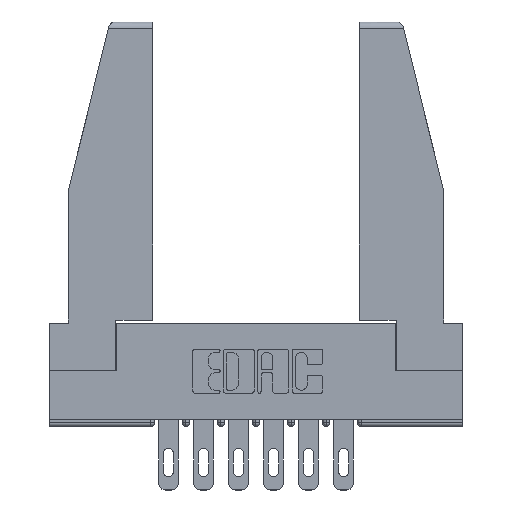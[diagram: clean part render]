
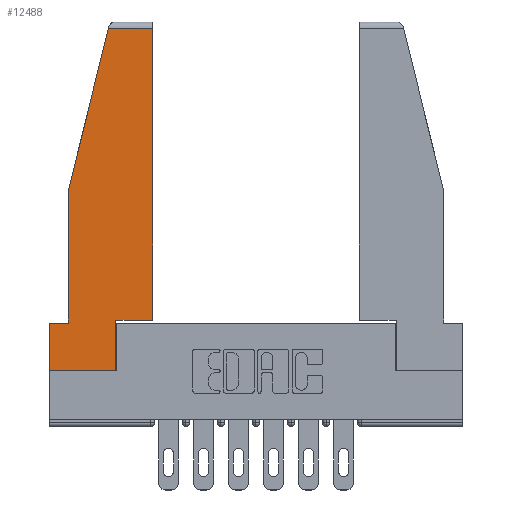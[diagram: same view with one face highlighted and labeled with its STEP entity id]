
A CAD part, top view. The second image highlights one B-rep face of the part: STEP entity #12488.
In plain terms, the highlighted planar face has unit normal (0, 0, 1).
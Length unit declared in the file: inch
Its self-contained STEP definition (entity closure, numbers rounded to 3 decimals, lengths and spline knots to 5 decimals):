
#52 = ORIENTED_EDGE ( 'NONE', *, *, #7661, .T. ) ;
#770 = LINE ( 'NONE', #2543, #12000 ) ;
#775 = DIRECTION ( 'NONE',  ( -1., 0., 0. ) ) ;
#874 = VECTOR ( 'NONE', #993, 39.37008 ) ;
#993 = DIRECTION ( 'NONE',  ( -0.239, -0.971, 0. ) ) ;
#1558 = VECTOR ( 'NONE', #3372, 39.37008 ) ;
#1620 = LINE ( 'NONE', #3783, #2023 ) ;
#1683 = DIRECTION ( 'NONE',  ( -1., 0., 0. ) ) ;
#1818 = DIRECTION ( 'NONE',  ( 1., 0., 0. ) ) ;
#1853 = CARTESIAN_POINT ( 'NONE',  ( 0., 0.21, 0. ) ) ;
#1905 = CARTESIAN_POINT ( 'NONE',  ( 0.271, 1.55, 0. ) ) ;
#2023 = VECTOR ( 'NONE', #9506, 39.37008 ) ;
#2178 = DIRECTION ( 'NONE',  ( 1., 0., 0. ) ) ;
#2543 = CARTESIAN_POINT ( 'NONE',  ( 0., 1.52, 0. ) ) ;
#2686 = ORIENTED_EDGE ( 'NONE', *, *, #4684, .T. ) ;
#2823 = CARTESIAN_POINT ( 'NONE',  ( 0.461, 1.52, 0. ) ) ;
#2955 = EDGE_CURVE ( 'NONE', #8437, #8369, #1620, .T. ) ;
#3372 = DIRECTION ( 'NONE',  ( 0., -1., 0. ) ) ;
#3496 = DIRECTION ( 'NONE',  ( 0., 1., 0. ) ) ;
#3629 = CARTESIAN_POINT ( 'NONE',  ( 0.461, 0.223, 0. ) ) ;
#3783 = CARTESIAN_POINT ( 'NONE',  ( 0.297, 0., 0. ) ) ;
#3878 = ORIENTED_EDGE ( 'NONE', *, *, #6867, .T. ) ;
#3941 = EDGE_CURVE ( 'NONE', #8189, #4542, #11826, .T. ) ;
#3943 = VERTEX_POINT ( 'NONE', #7784 ) ;
#4056 = EDGE_LOOP ( 'NONE', ( #52, #3878, #8968, #9953, #10837, #12380, #4109, #5168, #2686 ) ) ;
#4086 = EDGE_CURVE ( 'NONE', #3943, #8437, #10167, .T. ) ;
#4109 = ORIENTED_EDGE ( 'NONE', *, *, #4086, .T. ) ;
#4298 = LINE ( 'NONE', #7289, #1558 ) ;
#4358 = VERTEX_POINT ( 'NONE', #9883 ) ;
#4450 = CARTESIAN_POINT ( 'NONE',  ( 0.461, 0.223, 0. ) ) ;
#4542 = VERTEX_POINT ( 'NONE', #10339 ) ;
#4684 = EDGE_CURVE ( 'NONE', #8369, #11536, #12497, .T. ) ;
#4764 = CARTESIAN_POINT ( 'NONE',  ( 0.297, 0.223, 0. ) ) ;
#4903 = CARTESIAN_POINT ( 'NONE',  ( 0., 0., 0. ) ) ;
#5168 = ORIENTED_EDGE ( 'NONE', *, *, #2955, .T. ) ;
#5714 = VERTEX_POINT ( 'NONE', #2823 ) ;
#5809 = CARTESIAN_POINT ( 'NONE',  ( 0., 0.21, 0. ) ) ;
#6216 = CARTESIAN_POINT ( 'NONE',  ( 0.297, 0., 0. ) ) ;
#6316 = EDGE_CURVE ( 'NONE', #10459, #3943, #4298, .T. ) ;
#6600 = LINE ( 'NONE', #5809, #12125 ) ;
#6867 = EDGE_CURVE ( 'NONE', #5714, #8189, #770, .T. ) ;
#7289 = CARTESIAN_POINT ( 'NONE',  ( 0., 0.21, 0. ) ) ;
#7392 = VECTOR ( 'NONE', #9321, 39.37008 ) ;
#7661 = EDGE_CURVE ( 'NONE', #11536, #5714, #10514, .T. ) ;
#7742 = VECTOR ( 'NONE', #2178, 39.37008 ) ;
#7784 = CARTESIAN_POINT ( 'NONE',  ( 0., 0., 0. ) ) ;
#8039 = CARTESIAN_POINT ( 'NONE',  ( 0., 0., 0. ) ) ;
#8189 = VERTEX_POINT ( 'NONE', #10559 ) ;
#8352 = LINE ( 'NONE', #12319, #7392 ) ;
#8369 = VERTEX_POINT ( 'NONE', #10686 ) ;
#8437 = VERTEX_POINT ( 'NONE', #6216 ) ;
#8625 = EDGE_CURVE ( 'NONE', #4542, #4358, #8352, .T. ) ;
#8714 = DIRECTION ( 'NONE',  ( 1., 0., 0. ) ) ;
#8968 = ORIENTED_EDGE ( 'NONE', *, *, #3941, .T. ) ;
#9321 = DIRECTION ( 'NONE',  ( 0., -1., 0. ) ) ;
#9506 = DIRECTION ( 'NONE',  ( 0., 1., 0. ) ) ;
#9883 = CARTESIAN_POINT ( 'NONE',  ( 0.086, 0.21, 0. ) ) ;
#9953 = ORIENTED_EDGE ( 'NONE', *, *, #8625, .T. ) ;
#10167 = LINE ( 'NONE', #8039, #7742 ) ;
#10339 = CARTESIAN_POINT ( 'NONE',  ( 0.086, 0.8, 0. ) ) ;
#10459 = VERTEX_POINT ( 'NONE', #1853 ) ;
#10514 = LINE ( 'NONE', #3629, #10879 ) ;
#10559 = CARTESIAN_POINT ( 'NONE',  ( 0.2636, 1.52, 0. ) ) ;
#10686 = CARTESIAN_POINT ( 'NONE',  ( 0.297, 0.223, 0. ) ) ;
#10837 = ORIENTED_EDGE ( 'NONE', *, *, #12499, .T. ) ;
#10864 = AXIS2_PLACEMENT_3D ( 'NONE', #4903, #11798, #1818 ) ;
#10867 = VECTOR ( 'NONE', #8714, 39.37008 ) ;
#10879 = VECTOR ( 'NONE', #3496, 39.37008 ) ;
#11536 = VERTEX_POINT ( 'NONE', #4450 ) ;
#11663 = FACE_OUTER_BOUND ( 'NONE', #4056, .T. ) ;
#11798 = DIRECTION ( 'NONE',  ( 0., 0., 1. ) ) ;
#11826 = LINE ( 'NONE', #1905, #874 ) ;
#12000 = VECTOR ( 'NONE', #1683, 39.37008 ) ;
#12125 = VECTOR ( 'NONE', #775, 39.37008 ) ;
#12319 = CARTESIAN_POINT ( 'NONE',  ( 0.086, 0.8, 0. ) ) ;
#12380 = ORIENTED_EDGE ( 'NONE', *, *, #6316, .T. ) ;
#12488 = ADVANCED_FACE ( 'NONE', ( #11663 ), #12691, .T. ) ;
#12497 = LINE ( 'NONE', #4764, #10867 ) ;
#12499 = EDGE_CURVE ( 'NONE', #4358, #10459, #6600, .T. ) ;
#12691 = PLANE ( 'NONE',  #10864 ) ;
